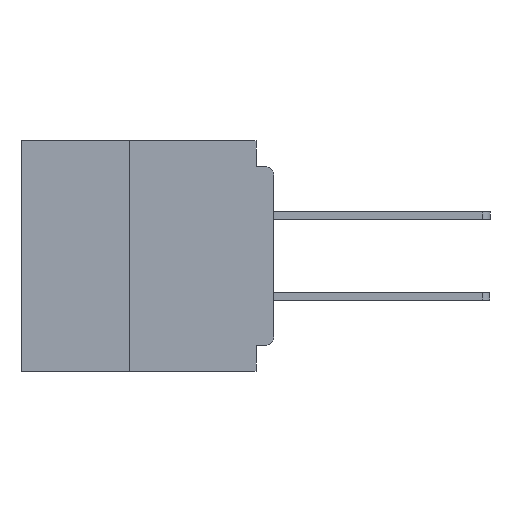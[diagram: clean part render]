
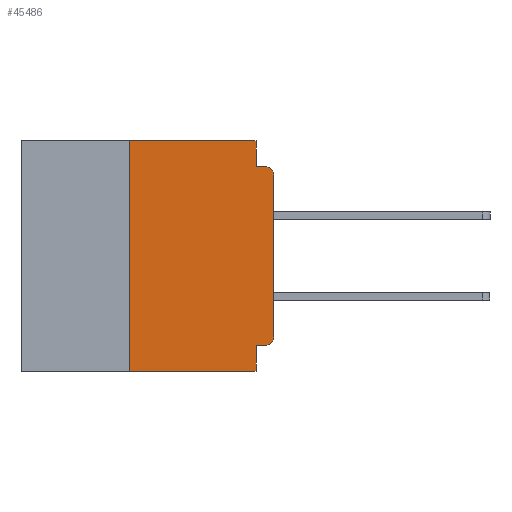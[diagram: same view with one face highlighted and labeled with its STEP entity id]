
A CAD part, left-side view. The second image highlights one B-rep face of the part: STEP entity #45486.
In plain terms, the highlighted planar face has unit normal (-1, 0, 0).
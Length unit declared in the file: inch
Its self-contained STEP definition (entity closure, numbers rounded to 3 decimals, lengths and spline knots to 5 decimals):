
#1333 = CARTESIAN_POINT ( 'NONE',  ( 0., 0.015, -0.06 ) ) ;
#1912 = ORIENTED_EDGE ( 'NONE', *, *, #40879, .F. ) ;
#2527 = VERTEX_POINT ( 'NONE', #52911 ) ;
#2742 = CARTESIAN_POINT ( 'NONE',  ( 0., 0.437, 0. ) ) ;
#2809 = ORIENTED_EDGE ( 'NONE', *, *, #51155, .T. ) ;
#3361 = VECTOR ( 'NONE', #50091, 39.37008 ) ;
#5472 = CARTESIAN_POINT ( 'NONE',  ( 0., 0.015, -0.34 ) ) ;
#5533 = DIRECTION ( 'NONE',  ( 0., 0., -1. ) ) ;
#5648 = VERTEX_POINT ( 'NONE', #35085 ) ;
#6314 = VECTOR ( 'NONE', #50189, 39.37008 ) ;
#7044 = CARTESIAN_POINT ( 'NONE',  ( 0., 0., 0. ) ) ;
#7980 = CARTESIAN_POINT ( 'NONE',  ( 0., 0., -0.06 ) ) ;
#8407 = VERTEX_POINT ( 'NONE', #20975 ) ;
#8417 = FACE_OUTER_BOUND ( 'NONE', #31581, .T. ) ;
#9191 = VERTEX_POINT ( 'NONE', #22149 ) ;
#9288 = AXIS2_PLACEMENT_3D ( 'NONE', #2742, #19362, #47770 ) ;
#9462 = CARTESIAN_POINT ( 'NONE',  ( 0., 0.25, -0.4 ) ) ;
#9590 = DIRECTION ( 'NONE',  ( 0., 0., -1. ) ) ;
#12195 = ORIENTED_EDGE ( 'NONE', *, *, #48768, .F. ) ;
#15404 = DIRECTION ( 'NONE',  ( 0., 0., -1. ) ) ;
#16194 = CARTESIAN_POINT ( 'NONE',  ( 0., 0., -0.045 ) ) ;
#17963 = DIRECTION ( 'NONE',  ( 0., -1., 0. ) ) ;
#18315 = VERTEX_POINT ( 'NONE', #7980 ) ;
#18947 = VERTEX_POINT ( 'NONE', #37895 ) ;
#19201 = ORIENTED_EDGE ( 'NONE', *, *, #49674, .T. ) ;
#19362 = DIRECTION ( 'NONE',  ( 1., 0., 0. ) ) ;
#19371 = EDGE_CURVE ( 'NONE', #5648, #8407, #50855, .T. ) ;
#20540 = ORIENTED_EDGE ( 'NONE', *, *, #19371, .F. ) ;
#20975 = CARTESIAN_POINT ( 'NONE',  ( 0., 0.031, -0.4 ) ) ;
#22149 = CARTESIAN_POINT ( 'NONE',  ( 0., 0.015, -0.045 ) ) ;
#23150 = VERTEX_POINT ( 'NONE', #49596 ) ;
#23280 = EDGE_CURVE ( 'NONE', #2527, #27370, #29754, .T. ) ;
#23841 = CIRCLE ( 'NONE', #24805, 0.015 ) ;
#24329 = DIRECTION ( 'NONE',  ( 0., 0., -1. ) ) ;
#24671 = VECTOR ( 'NONE', #31857, 39.37008 ) ;
#24805 = AXIS2_PLACEMENT_3D ( 'NONE', #1333, #30219, #5533 ) ;
#25108 = ORIENTED_EDGE ( 'NONE', *, *, #49555, .T. ) ;
#27069 = DIRECTION ( 'NONE',  ( 0., -1., 0. ) ) ;
#27370 = VERTEX_POINT ( 'NONE', #50366 ) ;
#28240 = LINE ( 'NONE', #43906, #48406 ) ;
#28463 = DIRECTION ( 'NONE',  ( 0., -1., 0. ) ) ;
#29407 = EDGE_CURVE ( 'NONE', #27370, #45059, #28240, .T. ) ;
#29754 = LINE ( 'NONE', #42378, #49919 ) ;
#30219 = DIRECTION ( 'NONE',  ( -1., 0., 0. ) ) ;
#31101 = VECTOR ( 'NONE', #27069, 39.37008 ) ;
#31581 = EDGE_LOOP ( 'NONE', ( #19201, #2809, #43791, #45115, #50499, #12195, #25108, #20540, #1912, #34114 ) ) ;
#31857 = DIRECTION ( 'NONE',  ( 0., 0., 1. ) ) ;
#34114 = ORIENTED_EDGE ( 'NONE', *, *, #51782, .T. ) ;
#34216 = DIRECTION ( 'NONE',  ( -1., 0., 0. ) ) ;
#34764 = VECTOR ( 'NONE', #28463, 39.37008 ) ;
#35085 = CARTESIAN_POINT ( 'NONE',  ( 0., 0.031, -0.355 ) ) ;
#35528 = LINE ( 'NONE', #7044, #24671 ) ;
#35652 = PLANE ( 'NONE',  #9288 ) ;
#36163 = LINE ( 'NONE', #9462, #3361 ) ;
#37786 = CIRCLE ( 'NONE', #39139, 0.015 ) ;
#37873 = CARTESIAN_POINT ( 'NONE',  ( 0., 0., -0.355 ) ) ;
#37895 = CARTESIAN_POINT ( 'NONE',  ( 0., 0.015, -0.355 ) ) ;
#39025 = LINE ( 'NONE', #37873, #6314 ) ;
#39139 = AXIS2_PLACEMENT_3D ( 'NONE', #5472, #34216, #9590 ) ;
#39410 = EDGE_CURVE ( 'NONE', #45059, #9191, #45471, .T. ) ;
#40879 = EDGE_CURVE ( 'NONE', #18947, #5648, #39025, .T. ) ;
#41420 = VECTOR ( 'NONE', #24329, 39.37008 ) ;
#42378 = CARTESIAN_POINT ( 'NONE',  ( 0., 0.437, 0. ) ) ;
#42561 = VERTEX_POINT ( 'NONE', #50236 ) ;
#43791 = ORIENTED_EDGE ( 'NONE', *, *, #39410, .F. ) ;
#43906 = CARTESIAN_POINT ( 'NONE',  ( 0., 0.031, 0. ) ) ;
#45006 = CARTESIAN_POINT ( 'NONE',  ( 0., 0.031, -0.045 ) ) ;
#45059 = VERTEX_POINT ( 'NONE', #45006 ) ;
#45115 = ORIENTED_EDGE ( 'NONE', *, *, #29407, .F. ) ;
#45471 = LINE ( 'NONE', #16194, #34764 ) ;
#45486 = ADVANCED_FACE ( 'NONE', ( #8417 ), #35652, .F. ) ;
#47770 = DIRECTION ( 'NONE',  ( 0., 0., -1. ) ) ;
#48406 = VECTOR ( 'NONE', #15404, 39.37008 ) ;
#48575 = CARTESIAN_POINT ( 'NONE',  ( 0., 0.031, -0.4 ) ) ;
#48768 = EDGE_CURVE ( 'NONE', #42561, #2527, #36163, .T. ) ;
#49555 = EDGE_CURVE ( 'NONE', #42561, #8407, #52523, .T. ) ;
#49596 = CARTESIAN_POINT ( 'NONE',  ( 0., 0., -0.34 ) ) ;
#49674 = EDGE_CURVE ( 'NONE', #23150, #18315, #35528, .T. ) ;
#49919 = VECTOR ( 'NONE', #17963, 39.37008 ) ;
#50091 = DIRECTION ( 'NONE',  ( 0., 0., 1. ) ) ;
#50189 = DIRECTION ( 'NONE',  ( 0., 1., 0. ) ) ;
#50236 = CARTESIAN_POINT ( 'NONE',  ( 0., 0.25, -0.4 ) ) ;
#50366 = CARTESIAN_POINT ( 'NONE',  ( 0., 0.031, 0. ) ) ;
#50499 = ORIENTED_EDGE ( 'NONE', *, *, #23280, .F. ) ;
#50855 = LINE ( 'NONE', #48575, #41420 ) ;
#51155 = EDGE_CURVE ( 'NONE', #18315, #9191, #23841, .T. ) ;
#51245 = CARTESIAN_POINT ( 'NONE',  ( 0., 0.437, -0.4 ) ) ;
#51782 = EDGE_CURVE ( 'NONE', #18947, #23150, #37786, .T. ) ;
#52523 = LINE ( 'NONE', #51245, #31101 ) ;
#52911 = CARTESIAN_POINT ( 'NONE',  ( 0., 0.25, 0. ) ) ;
